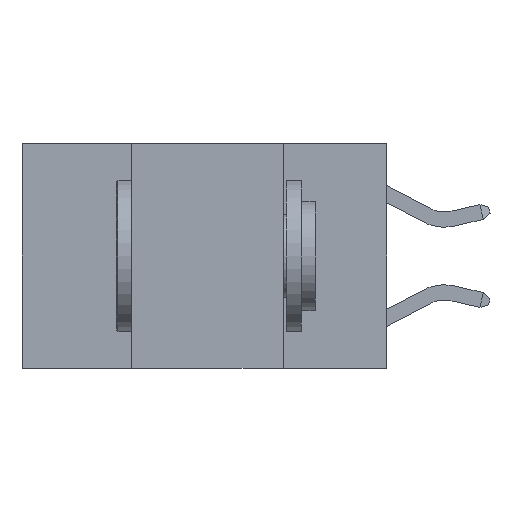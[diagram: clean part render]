
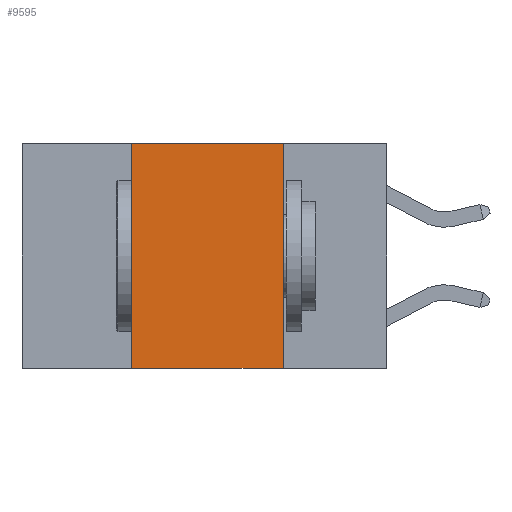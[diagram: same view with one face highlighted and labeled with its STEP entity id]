
A CAD part, left-side view. The second image highlights one B-rep face of the part: STEP entity #9595.
In plain terms, the highlighted planar face has unit normal (-1, 0, 0).
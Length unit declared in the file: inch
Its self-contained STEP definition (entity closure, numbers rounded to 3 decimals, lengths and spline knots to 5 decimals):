
#556 = CARTESIAN_POINT ( 'NONE',  ( 0., 0.6, 0. ) ) ;
#713 = DIRECTION ( 'NONE',  ( 0., 0., -1. ) ) ;
#1877 = VECTOR ( 'NONE', #21919, 39.37008 ) ;
#1897 = VECTOR ( 'NONE', #4601, 39.37008 ) ;
#2504 = LINE ( 'NONE', #12064, #1877 ) ;
#2677 = ORIENTED_EDGE ( 'NONE', *, *, #3163, .F. ) ;
#3163 = EDGE_CURVE ( 'NONE', #9719, #12559, #15592, .T. ) ;
#4601 = DIRECTION ( 'NONE',  ( 0., 0., 1. ) ) ;
#5480 = DIRECTION ( 'NONE',  ( 1., 0., 0. ) ) ;
#6427 = VECTOR ( 'NONE', #9301, 39.37008 ) ;
#6450 = ORIENTED_EDGE ( 'NONE', *, *, #16685, .T. ) ;
#8317 = VERTEX_POINT ( 'NONE', #15505 ) ;
#8502 = CARTESIAN_POINT ( 'NONE',  ( 0., 0.42, 0. ) ) ;
#9059 = AXIS2_PLACEMENT_3D ( 'NONE', #556, #5480, #713 ) ;
#9219 = ORIENTED_EDGE ( 'NONE', *, *, #24209, .F. ) ;
#9301 = DIRECTION ( 'NONE',  ( 0., -1., 0. ) ) ;
#9595 = ADVANCED_FACE ( 'NONE', ( #12673 ), #22371, .F. ) ;
#9719 = VERTEX_POINT ( 'NONE', #8502 ) ;
#12064 = CARTESIAN_POINT ( 'NONE',  ( 0., 0.17, 0. ) ) ;
#12559 = VERTEX_POINT ( 'NONE', #14616 ) ;
#12673 = FACE_OUTER_BOUND ( 'NONE', #27565, .T. ) ;
#14616 = CARTESIAN_POINT ( 'NONE',  ( 0., 0.17, 0. ) ) ;
#14715 = LINE ( 'NONE', #16780, #6427 ) ;
#15505 = CARTESIAN_POINT ( 'NONE',  ( 0., 0.42, -0.37 ) ) ;
#15592 = LINE ( 'NONE', #20378, #30010 ) ;
#16685 = EDGE_CURVE ( 'NONE', #8317, #17607, #14715, .T. ) ;
#16780 = CARTESIAN_POINT ( 'NONE',  ( 0., 0.6, -0.37 ) ) ;
#17607 = VERTEX_POINT ( 'NONE', #27943 ) ;
#18615 = CARTESIAN_POINT ( 'NONE',  ( 0., 0.42, 0. ) ) ;
#19920 = DIRECTION ( 'NONE',  ( 0., -1., 0. ) ) ;
#20378 = CARTESIAN_POINT ( 'NONE',  ( 0., 0.6, 0. ) ) ;
#21919 = DIRECTION ( 'NONE',  ( 0., 0., -1. ) ) ;
#22371 = PLANE ( 'NONE',  #9059 ) ;
#22966 = ORIENTED_EDGE ( 'NONE', *, *, #28364, .F. ) ;
#24209 = EDGE_CURVE ( 'NONE', #8317, #9719, #28983, .T. ) ;
#27565 = EDGE_LOOP ( 'NONE', ( #22966, #2677, #9219, #6450 ) ) ;
#27943 = CARTESIAN_POINT ( 'NONE',  ( 0., 0.17, -0.37 ) ) ;
#28364 = EDGE_CURVE ( 'NONE', #12559, #17607, #2504, .T. ) ;
#28983 = LINE ( 'NONE', #18615, #1897 ) ;
#30010 = VECTOR ( 'NONE', #19920, 39.37008 ) ;
